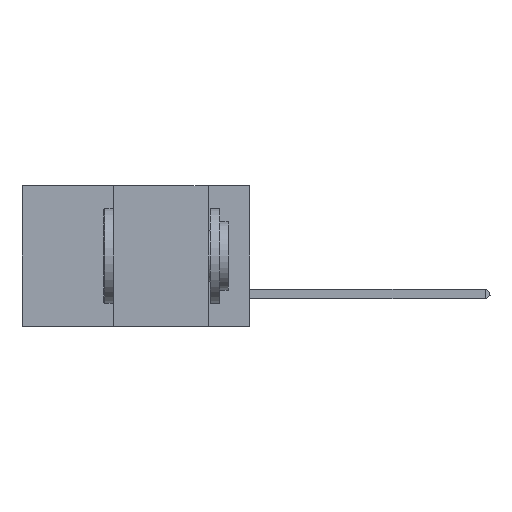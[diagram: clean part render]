
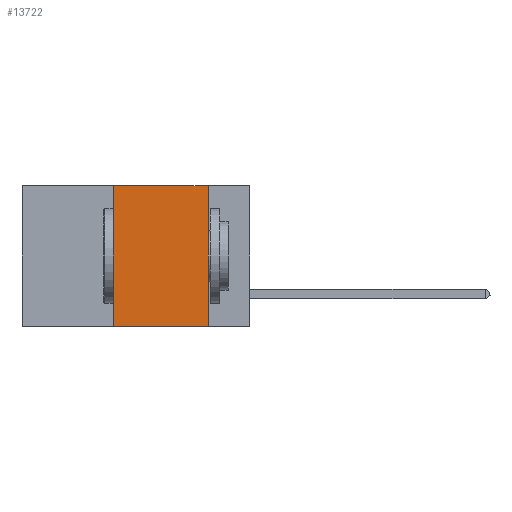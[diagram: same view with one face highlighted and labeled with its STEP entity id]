
A CAD part, left-side view. The second image highlights one B-rep face of the part: STEP entity #13722.
In plain terms, the highlighted planar face has unit normal (-1, 0, 0).
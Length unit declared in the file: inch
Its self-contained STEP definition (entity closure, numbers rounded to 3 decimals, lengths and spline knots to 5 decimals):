
#188 = VECTOR ( 'NONE', #2037, 39.37008 ) ;
#772 = FACE_OUTER_BOUND ( 'NONE', #2366, .T. ) ;
#962 = VERTEX_POINT ( 'NONE', #15577 ) ;
#1303 = LINE ( 'NONE', #6558, #11347 ) ;
#2037 = DIRECTION ( 'NONE',  ( 0., -1., 0. ) ) ;
#2057 = VECTOR ( 'NONE', #13876, 39.37008 ) ;
#2366 = EDGE_LOOP ( 'NONE', ( #19200, #14063, #15232, #10480 ) ) ;
#4217 = CARTESIAN_POINT ( 'NONE',  ( 0., 0.6, 0. ) ) ;
#4425 = CARTESIAN_POINT ( 'NONE',  ( 0., 0.36, 0. ) ) ;
#5650 = CARTESIAN_POINT ( 'NONE',  ( 0., 0.36, -0.37 ) ) ;
#6237 = VERTEX_POINT ( 'NONE', #8647 ) ;
#6377 = LINE ( 'NONE', #12205, #2057 ) ;
#6558 = CARTESIAN_POINT ( 'NONE',  ( 0., 0.36, 0. ) ) ;
#6996 = EDGE_CURVE ( 'NONE', #6237, #962, #6377, .T. ) ;
#8647 = CARTESIAN_POINT ( 'NONE',  ( 0., 0.11, 0. ) ) ;
#8927 = PLANE ( 'NONE',  #20161 ) ;
#9273 = LINE ( 'NONE', #16958, #188 ) ;
#10480 = ORIENTED_EDGE ( 'NONE', *, *, #11767, .T. ) ;
#10987 = VERTEX_POINT ( 'NONE', #5650 ) ;
#11347 = VECTOR ( 'NONE', #16828, 39.37008 ) ;
#11767 = EDGE_CURVE ( 'NONE', #10987, #962, #19019, .T. ) ;
#12205 = CARTESIAN_POINT ( 'NONE',  ( 0., 0.11, 0. ) ) ;
#13722 = ADVANCED_FACE ( 'NONE', ( #772 ), #8927, .F. ) ;
#13876 = DIRECTION ( 'NONE',  ( 0., 0., -1. ) ) ;
#14063 = ORIENTED_EDGE ( 'NONE', *, *, #14557, .F. ) ;
#14557 = EDGE_CURVE ( 'NONE', #18968, #6237, #9273, .T. ) ;
#15232 = ORIENTED_EDGE ( 'NONE', *, *, #18779, .F. ) ;
#15521 = DIRECTION ( 'NONE',  ( 1., 0., 0. ) ) ;
#15577 = CARTESIAN_POINT ( 'NONE',  ( 0., 0.11, -0.37 ) ) ;
#15648 = DIRECTION ( 'NONE',  ( 0., 0., -1. ) ) ;
#16828 = DIRECTION ( 'NONE',  ( 0., 0., 1. ) ) ;
#16958 = CARTESIAN_POINT ( 'NONE',  ( 0., 0.6, 0. ) ) ;
#18779 = EDGE_CURVE ( 'NONE', #10987, #18968, #1303, .T. ) ;
#18968 = VERTEX_POINT ( 'NONE', #4425 ) ;
#18985 = DIRECTION ( 'NONE',  ( 0., -1., 0. ) ) ;
#19019 = LINE ( 'NONE', #20783, #19261 ) ;
#19200 = ORIENTED_EDGE ( 'NONE', *, *, #6996, .F. ) ;
#19261 = VECTOR ( 'NONE', #18985, 39.37008 ) ;
#20161 = AXIS2_PLACEMENT_3D ( 'NONE', #4217, #15521, #15648 ) ;
#20783 = CARTESIAN_POINT ( 'NONE',  ( 0., 0.6, -0.37 ) ) ;
